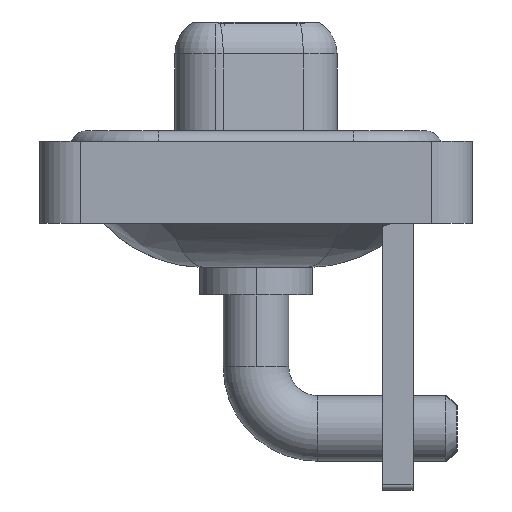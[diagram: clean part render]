
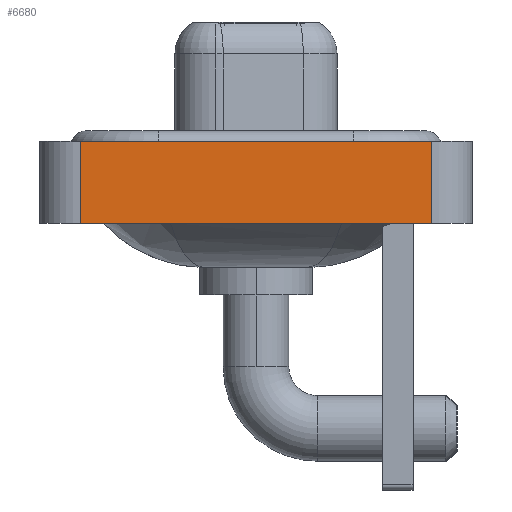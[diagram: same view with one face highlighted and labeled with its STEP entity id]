
A CAD part, left-side view. The second image highlights one B-rep face of the part: STEP entity #6680.
In plain terms, the highlighted planar face has unit normal (-1, 0, 0).
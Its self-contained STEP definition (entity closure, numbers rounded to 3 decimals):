
#748 = LINE ( 'NONE', #15669, #9162 ) ;
#1178 = LINE ( 'NONE', #8022, #1488 ) ;
#1199 = VERTEX_POINT ( 'NONE', #7916 ) ;
#1488 = VECTOR ( 'NONE', #8194, 1000. ) ;
#1972 = EDGE_CURVE ( 'NONE', #1199, #3382, #748, .T. ) ;
#2714 = DIRECTION ( 'NONE',  ( 0., 0., 1. ) ) ;
#2865 = FACE_OUTER_BOUND ( 'NONE', #17213, .T. ) ;
#2963 = CARTESIAN_POINT ( 'NONE',  ( -7.25, -8.55, -3.6 ) ) ;
#3382 = VERTEX_POINT ( 'NONE', #10333 ) ;
#4808 = DIRECTION ( 'NONE',  ( 0., 0., 1. ) ) ;
#6093 = CARTESIAN_POINT ( 'NONE',  ( -7.25, -8.55, -3.6 ) ) ;
#6454 = ORIENTED_EDGE ( 'NONE', *, *, #10518, .T. ) ;
#6680 = ADVANCED_FACE ( 'NONE', ( #2865 ), #8350, .T. ) ;
#7003 = DIRECTION ( 'NONE',  ( -1., 0., 0. ) ) ;
#7916 = CARTESIAN_POINT ( 'NONE',  ( -7.25, 8.55, -3.6 ) ) ;
#8022 = CARTESIAN_POINT ( 'NONE',  ( -7.25, -8.55, 0.4 ) ) ;
#8194 = DIRECTION ( 'NONE',  ( 0., -1., 0. ) ) ;
#8350 = PLANE ( 'NONE',  #15108 ) ;
#9007 = VECTOR ( 'NONE', #13835, 1000. ) ;
#9162 = VECTOR ( 'NONE', #4808, 1000. ) ;
#9353 = VERTEX_POINT ( 'NONE', #6093 ) ;
#9533 = CARTESIAN_POINT ( 'NONE',  ( -7.25, -8.55, -3.6 ) ) ;
#9953 = CARTESIAN_POINT ( 'NONE',  ( -7.25, -8.55, 0.4 ) ) ;
#10333 = CARTESIAN_POINT ( 'NONE',  ( -7.25, 8.55, 0.4 ) ) ;
#10518 = EDGE_CURVE ( 'NONE', #9353, #11845, #13482, .T. ) ;
#10567 = EDGE_CURVE ( 'NONE', #3382, #11845, #1178, .T. ) ;
#11136 = LINE ( 'NONE', #2963, #9007 ) ;
#11845 = VERTEX_POINT ( 'NONE', #9953 ) ;
#12472 = DIRECTION ( 'NONE',  ( 0., 0., 1. ) ) ;
#13164 = EDGE_CURVE ( 'NONE', #1199, #9353, #11136, .T. ) ;
#13482 = LINE ( 'NONE', #9533, #17286 ) ;
#13818 = CARTESIAN_POINT ( 'NONE',  ( -7.25, -8.55, -3.6 ) ) ;
#13835 = DIRECTION ( 'NONE',  ( 0., -1., 0. ) ) ;
#14091 = ORIENTED_EDGE ( 'NONE', *, *, #1972, .F. ) ;
#14852 = ORIENTED_EDGE ( 'NONE', *, *, #10567, .F. ) ;
#15108 = AXIS2_PLACEMENT_3D ( 'NONE', #13818, #7003, #12472 ) ;
#15669 = CARTESIAN_POINT ( 'NONE',  ( -7.25, 8.55, -3.6 ) ) ;
#17213 = EDGE_LOOP ( 'NONE', ( #6454, #14852, #14091, #17414 ) ) ;
#17286 = VECTOR ( 'NONE', #2714, 1000. ) ;
#17414 = ORIENTED_EDGE ( 'NONE', *, *, #13164, .T. ) ;
